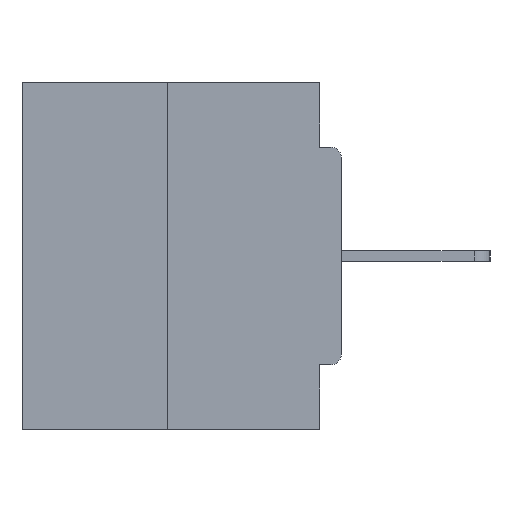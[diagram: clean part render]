
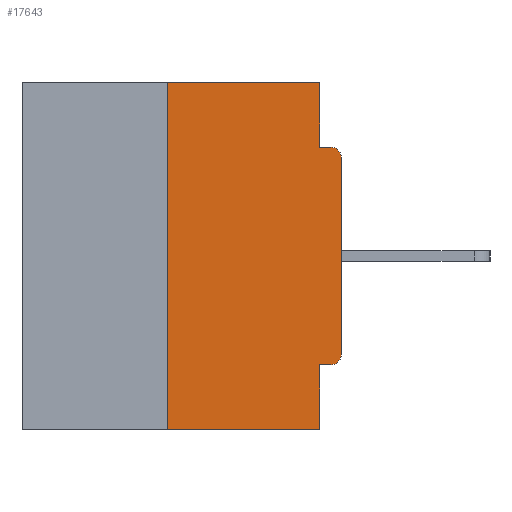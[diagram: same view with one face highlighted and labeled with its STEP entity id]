
A CAD part, left-side view. The second image highlights one B-rep face of the part: STEP entity #17643.
In plain terms, the highlighted planar face has unit normal (-1, 0, 0).
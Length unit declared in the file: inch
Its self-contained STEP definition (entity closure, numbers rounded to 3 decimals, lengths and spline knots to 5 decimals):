
#57 = DIRECTION ( 'NONE',  ( 0., 0., -1. ) ) ;
#75 = VERTEX_POINT ( 'NONE', #16390 ) ;
#1406 = DIRECTION ( 'NONE',  ( 0., -1., 0. ) ) ;
#1502 = VERTEX_POINT ( 'NONE', #10968 ) ;
#1578 = FACE_OUTER_BOUND ( 'NONE', #5191, .T. ) ;
#1624 = AXIS2_PLACEMENT_3D ( 'NONE', #18310, #27829, #11501 ) ;
#1714 = DIRECTION ( 'NONE',  ( 0., -1., 0. ) ) ;
#2322 = VECTOR ( 'NONE', #1406, 39.37008 ) ;
#2536 = CARTESIAN_POINT ( 'NONE',  ( 0., 0.031, 0. ) ) ;
#3696 = ORIENTED_EDGE ( 'NONE', *, *, #6279, .F. ) ;
#4472 = DIRECTION ( 'NONE',  ( 0., 0., -1. ) ) ;
#4823 = VERTEX_POINT ( 'NONE', #2536 ) ;
#5031 = VERTEX_POINT ( 'NONE', #10986 ) ;
#5191 = EDGE_LOOP ( 'NONE', ( #7360, #9067, #10156, #27784, #3696, #27661, #5945, #14764, #19456, #23585 ) ) ;
#5343 = LINE ( 'NONE', #7738, #24974 ) ;
#5692 = DIRECTION ( 'NONE',  ( 0., 0., 1. ) ) ;
#5945 = ORIENTED_EDGE ( 'NONE', *, *, #14569, .T. ) ;
#5980 = LINE ( 'NONE', #21865, #11875 ) ;
#6243 = CARTESIAN_POINT ( 'NONE',  ( 0., 0., -0.0935 ) ) ;
#6279 = EDGE_CURVE ( 'NONE', #14993, #24081, #15131, .T. ) ;
#6371 = VERTEX_POINT ( 'NONE', #14601 ) ;
#6560 = LINE ( 'NONE', #20327, #18081 ) ;
#6979 = AXIS2_PLACEMENT_3D ( 'NONE', #14704, #12280, #8044 ) ;
#7360 = ORIENTED_EDGE ( 'NONE', *, *, #11498, .F. ) ;
#7738 = CARTESIAN_POINT ( 'NONE',  ( 0., 0.031, -0.5 ) ) ;
#7762 = LINE ( 'NONE', #12763, #19935 ) ;
#8044 = DIRECTION ( 'NONE',  ( 0., 0., -1. ) ) ;
#8233 = DIRECTION ( 'NONE',  ( 1., 0., 0. ) ) ;
#8320 = VECTOR ( 'NONE', #10989, 39.37008 ) ;
#8458 = CARTESIAN_POINT ( 'NONE',  ( 0., 0.015, -0.4065 ) ) ;
#9067 = ORIENTED_EDGE ( 'NONE', *, *, #9778, .F. ) ;
#9778 = EDGE_CURVE ( 'NONE', #5031, #6371, #13708, .T. ) ;
#10100 = VERTEX_POINT ( 'NONE', #26108 ) ;
#10156 = ORIENTED_EDGE ( 'NONE', *, *, #13005, .T. ) ;
#10793 = PLANE ( 'NONE',  #26051 ) ;
#10968 = CARTESIAN_POINT ( 'NONE',  ( 0., 0.031, -0.5 ) ) ;
#10986 = CARTESIAN_POINT ( 'NONE',  ( 0., 0.25, -0.5 ) ) ;
#10989 = DIRECTION ( 'NONE',  ( 0., 0., 1. ) ) ;
#11498 = EDGE_CURVE ( 'NONE', #6371, #4823, #7762, .T. ) ;
#11501 = DIRECTION ( 'NONE',  ( 0., 0., -1. ) ) ;
#11770 = CIRCLE ( 'NONE', #1624, 0.015 ) ;
#11875 = VECTOR ( 'NONE', #5692, 39.37008 ) ;
#12210 = EDGE_CURVE ( 'NONE', #75, #10100, #11770, .T. ) ;
#12280 = DIRECTION ( 'NONE',  ( -1., 0., 0. ) ) ;
#12763 = CARTESIAN_POINT ( 'NONE',  ( 0., 0.46, 0. ) ) ;
#13005 = EDGE_CURVE ( 'NONE', #5031, #1502, #6560, .T. ) ;
#13307 = EDGE_CURVE ( 'NONE', #14993, #18378, #15183, .T. ) ;
#13672 = VERTEX_POINT ( 'NONE', #19212 ) ;
#13708 = LINE ( 'NONE', #29455, #8320 ) ;
#14569 = EDGE_CURVE ( 'NONE', #18378, #75, #5980, .T. ) ;
#14601 = CARTESIAN_POINT ( 'NONE',  ( 0., 0.25, 0. ) ) ;
#14704 = CARTESIAN_POINT ( 'NONE',  ( 0., 0.015, -0.3915 ) ) ;
#14764 = ORIENTED_EDGE ( 'NONE', *, *, #12210, .T. ) ;
#14993 = VERTEX_POINT ( 'NONE', #8458 ) ;
#15131 = LINE ( 'NONE', #26931, #15583 ) ;
#15183 = CIRCLE ( 'NONE', #6979, 0.015 ) ;
#15583 = VECTOR ( 'NONE', #20824, 39.37008 ) ;
#15885 = CARTESIAN_POINT ( 'NONE',  ( 0., 0.031, -0.4065 ) ) ;
#15962 = DIRECTION ( 'NONE',  ( 0., 0., -1. ) ) ;
#16280 = VECTOR ( 'NONE', #15962, 39.37008 ) ;
#16390 = CARTESIAN_POINT ( 'NONE',  ( 0., 0., -0.1085 ) ) ;
#17271 = EDGE_CURVE ( 'NONE', #4823, #13672, #27169, .T. ) ;
#17305 = DIRECTION ( 'NONE',  ( 0., -1., 0. ) ) ;
#17643 = ADVANCED_FACE ( 'NONE', ( #1578 ), #10793, .F. ) ;
#17887 = LINE ( 'NONE', #6243, #2322 ) ;
#18081 = VECTOR ( 'NONE', #1714, 39.37008 ) ;
#18252 = CARTESIAN_POINT ( 'NONE',  ( 0., 0.031, 0. ) ) ;
#18310 = CARTESIAN_POINT ( 'NONE',  ( 0., 0.015, -0.1085 ) ) ;
#18378 = VERTEX_POINT ( 'NONE', #26737 ) ;
#19212 = CARTESIAN_POINT ( 'NONE',  ( 0., 0.031, -0.0935 ) ) ;
#19456 = ORIENTED_EDGE ( 'NONE', *, *, #26950, .F. ) ;
#19935 = VECTOR ( 'NONE', #17305, 39.37008 ) ;
#20030 = CARTESIAN_POINT ( 'NONE',  ( 0., 0.46, 0. ) ) ;
#20327 = CARTESIAN_POINT ( 'NONE',  ( 0., 0.46, -0.5 ) ) ;
#20824 = DIRECTION ( 'NONE',  ( 0., 1., 0. ) ) ;
#21865 = CARTESIAN_POINT ( 'NONE',  ( 0., 0., 0. ) ) ;
#23585 = ORIENTED_EDGE ( 'NONE', *, *, #17271, .F. ) ;
#23800 = EDGE_CURVE ( 'NONE', #24081, #1502, #5343, .T. ) ;
#24081 = VERTEX_POINT ( 'NONE', #15885 ) ;
#24974 = VECTOR ( 'NONE', #4472, 39.37008 ) ;
#26051 = AXIS2_PLACEMENT_3D ( 'NONE', #20030, #8233, #57 ) ;
#26108 = CARTESIAN_POINT ( 'NONE',  ( 0., 0.015, -0.0935 ) ) ;
#26737 = CARTESIAN_POINT ( 'NONE',  ( 0., 0., -0.3915 ) ) ;
#26931 = CARTESIAN_POINT ( 'NONE',  ( 0., 0., -0.4065 ) ) ;
#26950 = EDGE_CURVE ( 'NONE', #13672, #10100, #17887, .T. ) ;
#27169 = LINE ( 'NONE', #18252, #16280 ) ;
#27661 = ORIENTED_EDGE ( 'NONE', *, *, #13307, .T. ) ;
#27784 = ORIENTED_EDGE ( 'NONE', *, *, #23800, .F. ) ;
#27829 = DIRECTION ( 'NONE',  ( -1., 0., 0. ) ) ;
#29455 = CARTESIAN_POINT ( 'NONE',  ( 0., 0.25, 0. ) ) ;
